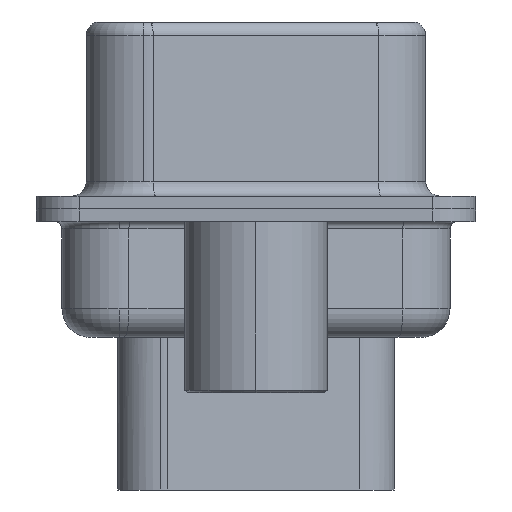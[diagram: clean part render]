
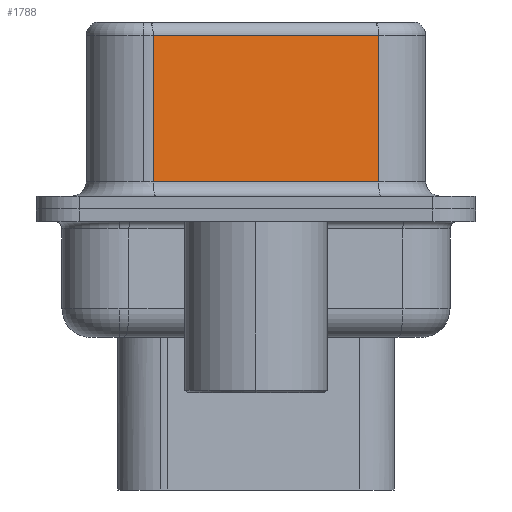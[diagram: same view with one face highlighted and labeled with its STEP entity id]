
A CAD part, left-side view. The second image highlights one B-rep face of the part: STEP entity #1788.
In plain terms, the highlighted planar face has unit normal (-0.985, -0.174, 0).
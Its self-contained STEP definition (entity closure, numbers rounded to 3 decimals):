
#1788 = ADVANCED_FACE ( 'NONE', ( #16370 ), #16524, .F. ) ;
#2703 = CARTESIAN_POINT ( 'NONE',  ( 3.735, 3.603, 6.07 ) ) ;
#3219 = VECTOR ( 'NONE', #21573, 1000. ) ;
#3326 = VECTOR ( 'NONE', #6261, 1000. ) ;
#4769 = EDGE_CURVE ( 'NONE', #26818, #25409, #6364, .T. ) ;
#5912 = EDGE_LOOP ( 'NONE', ( #17344, #30787, #22225, #11333 ) ) ;
#6261 = DIRECTION ( 'NONE',  ( 0., 0., -1. ) ) ;
#6364 = LINE ( 'NONE', #23814, #18254 ) ;
#8517 = CARTESIAN_POINT ( 'NONE',  ( 3.735, 3.603, 0.95 ) ) ;
#9011 = CARTESIAN_POINT ( 'NONE',  ( 5.128, -4.297, 6.07 ) ) ;
#11333 = ORIENTED_EDGE ( 'NONE', *, *, #4769, .T. ) ;
#13431 = DIRECTION ( 'NONE',  ( -0.174, 0.985, 0. ) ) ;
#15879 = CARTESIAN_POINT ( 'NONE',  ( 5.128, -4.297, 6.57 ) ) ;
#16036 = CARTESIAN_POINT ( 'NONE',  ( 5.128, -4.297, 6.57 ) ) ;
#16370 = FACE_OUTER_BOUND ( 'NONE', #5912, .T. ) ;
#16524 = PLANE ( 'NONE',  #31609 ) ;
#17344 = ORIENTED_EDGE ( 'NONE', *, *, #22197, .F. ) ;
#17465 = VERTEX_POINT ( 'NONE', #29303 ) ;
#18254 = VECTOR ( 'NONE', #31366, 1000. ) ;
#21573 = DIRECTION ( 'NONE',  ( -0.174, 0.985, 0. ) ) ;
#21834 = EDGE_CURVE ( 'NONE', #29261, #26818, #26864, .T. ) ;
#22197 = EDGE_CURVE ( 'NONE', #17465, #25409, #28473, .T. ) ;
#22225 = ORIENTED_EDGE ( 'NONE', *, *, #21834, .T. ) ;
#23814 = CARTESIAN_POINT ( 'NONE',  ( 5.128, -4.297, 0.95 ) ) ;
#24023 = LINE ( 'NONE', #9011, #3219 ) ;
#24403 = DIRECTION ( 'NONE',  ( 0., 0., -1. ) ) ;
#25409 = VERTEX_POINT ( 'NONE', #25592 ) ;
#25592 = CARTESIAN_POINT ( 'NONE',  ( 5.128, -4.297, 0.95 ) ) ;
#26342 = DIRECTION ( 'NONE',  ( 0.985, 0.174, 0. ) ) ;
#26697 = CARTESIAN_POINT ( 'NONE',  ( 3.735, 3.603, 6.57 ) ) ;
#26818 = VERTEX_POINT ( 'NONE', #8517 ) ;
#26864 = LINE ( 'NONE', #26697, #28876 ) ;
#28473 = LINE ( 'NONE', #16036, #3326 ) ;
#28876 = VECTOR ( 'NONE', #24403, 1000. ) ;
#29261 = VERTEX_POINT ( 'NONE', #2703 ) ;
#29303 = CARTESIAN_POINT ( 'NONE',  ( 5.128, -4.297, 6.07 ) ) ;
#29703 = EDGE_CURVE ( 'NONE', #17465, #29261, #24023, .T. ) ;
#30787 = ORIENTED_EDGE ( 'NONE', *, *, #29703, .T. ) ;
#31366 = DIRECTION ( 'NONE',  ( 0.174, -0.985, 0. ) ) ;
#31609 = AXIS2_PLACEMENT_3D ( 'NONE', #15879, #26342, #13431 ) ;
